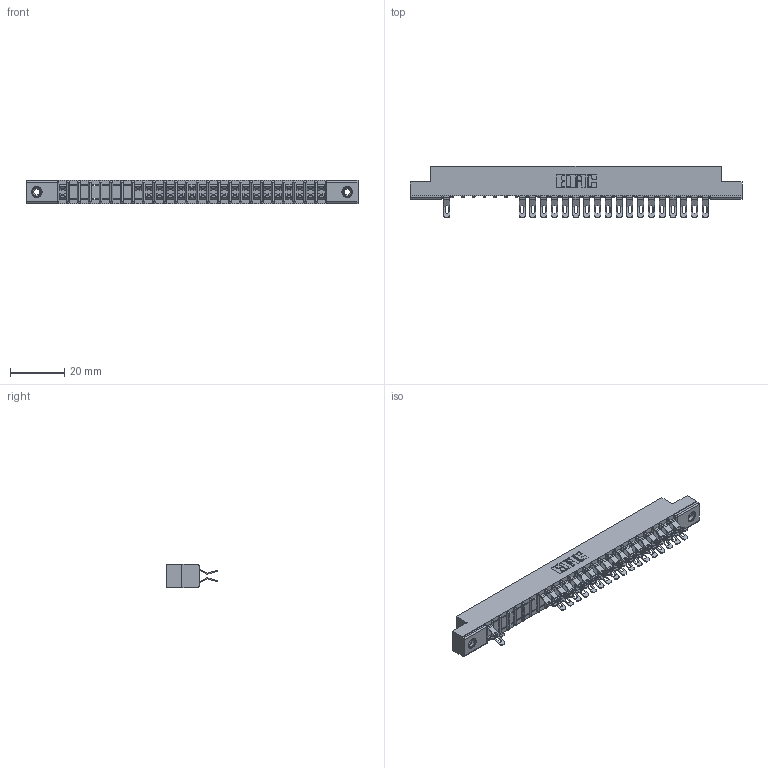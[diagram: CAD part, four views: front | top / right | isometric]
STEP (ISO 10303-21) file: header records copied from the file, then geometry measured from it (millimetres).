
FILE_DESCRIPTION (( 'STEP AP203' ), '1' );
FILE_NAME ('307-050-555-208.STEP', '2018-08-06T04:38:18', ( '' ), ( '' ), 'SwSTEP 2.0', 'SolidWorks 2016', '' );
FILE_SCHEMA (( 'CONFIG_CONTROL_DESIGN' ));
Length unit declared in the file: inch
Products named in the file (4): 307-290-001_555; 345-250-001_345-250-003-102; 307-050-555-208; 307 Part_.156 Dia Mounting Holes
Assembly tree (40 placements, depth 2):
  307-050-555-208
    307 Part_.156 Dia Mounting Holes
    307-290-001_555  x37
    345-250-001_345-250-003-102  x2
Bounding box: 122.07 x 18.75 x 8.71 mm (x, y, z)
Volume: 7919.9 mm3; surface area: 13781.5 mm2
Topology: 40 solids, 40 shells, 2591 faces, 7572 edges, 4920 vertices
Faces by surface type: plane 1438, cylinder 1085, sphere 52, cone 12, torus 4
Entity records: 25634 total; most frequent: CARTESIAN_POINT 4243, ORIENTED_EDGE 4212, DIRECTION 4166, EDGE_CURVE 2106, VECTOR 1596, LINE 1596, VERTEX_POINT 1362, AXIS2_PLACEMENT_3D 1285
